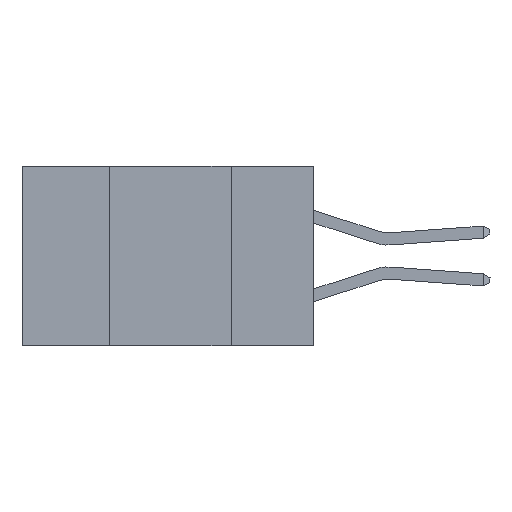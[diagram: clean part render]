
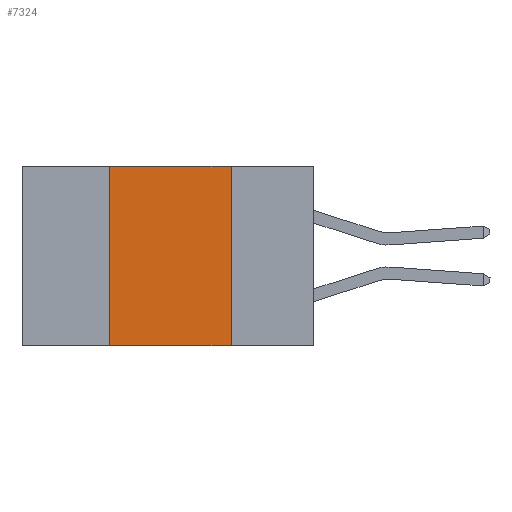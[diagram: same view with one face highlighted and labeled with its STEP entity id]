
A CAD part, left-side view. The second image highlights one B-rep face of the part: STEP entity #7324.
In plain terms, the highlighted planar face has unit normal (-1, 0, 0).
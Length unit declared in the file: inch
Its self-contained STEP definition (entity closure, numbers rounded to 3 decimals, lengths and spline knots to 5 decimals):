
#58 = CARTESIAN_POINT ( 'NONE',  ( 0., 0.42, 0. ) ) ;
#336 = CARTESIAN_POINT ( 'NONE',  ( 0., 0.42, -0.37 ) ) ;
#539 = DIRECTION ( 'NONE',  ( 0., 0., -1. ) ) ;
#818 = AXIS2_PLACEMENT_3D ( 'NONE', #9331, #6070, #539 ) ;
#955 = LINE ( 'NONE', #58, #3786 ) ;
#1066 = EDGE_CURVE ( 'NONE', #6573, #5884, #3466, .T. ) ;
#1088 = DIRECTION ( 'NONE',  ( 0., 0., 1. ) ) ;
#1171 = VERTEX_POINT ( 'NONE', #3477 ) ;
#3031 = EDGE_LOOP ( 'NONE', ( #5672, #8252, #6596, #4753 ) ) ;
#3214 = VECTOR ( 'NONE', #9567, 39.37008 ) ;
#3466 = LINE ( 'NONE', #7204, #5532 ) ;
#3477 = CARTESIAN_POINT ( 'NONE',  ( 0., 0.17, 0. ) ) ;
#3499 = DIRECTION ( 'NONE',  ( 0., -1., 0. ) ) ;
#3786 = VECTOR ( 'NONE', #1088, 39.37008 ) ;
#4381 = DIRECTION ( 'NONE',  ( 0., -1., 0. ) ) ;
#4454 = LINE ( 'NONE', #9964, #8628 ) ;
#4753 = ORIENTED_EDGE ( 'NONE', *, *, #1066, .T. ) ;
#5532 = VECTOR ( 'NONE', #3499, 39.37008 ) ;
#5593 = EDGE_CURVE ( 'NONE', #5878, #1171, #4454, .T. ) ;
#5672 = ORIENTED_EDGE ( 'NONE', *, *, #9270, .F. ) ;
#5878 = VERTEX_POINT ( 'NONE', #8434 ) ;
#5884 = VERTEX_POINT ( 'NONE', #9475 ) ;
#6070 = DIRECTION ( 'NONE',  ( 1., 0., 0. ) ) ;
#6573 = VERTEX_POINT ( 'NONE', #336 ) ;
#6596 = ORIENTED_EDGE ( 'NONE', *, *, #10728, .F. ) ;
#7204 = CARTESIAN_POINT ( 'NONE',  ( 0., 0.6, -0.37 ) ) ;
#7324 = ADVANCED_FACE ( 'NONE', ( #8849 ), #10783, .F. ) ;
#7532 = LINE ( 'NONE', #8747, #3214 ) ;
#8252 = ORIENTED_EDGE ( 'NONE', *, *, #5593, .F. ) ;
#8434 = CARTESIAN_POINT ( 'NONE',  ( 0., 0.42, 0. ) ) ;
#8628 = VECTOR ( 'NONE', #4381, 39.37008 ) ;
#8747 = CARTESIAN_POINT ( 'NONE',  ( 0., 0.17, 0. ) ) ;
#8849 = FACE_OUTER_BOUND ( 'NONE', #3031, .T. ) ;
#9270 = EDGE_CURVE ( 'NONE', #1171, #5884, #7532, .T. ) ;
#9331 = CARTESIAN_POINT ( 'NONE',  ( 0., 0.6, 0. ) ) ;
#9475 = CARTESIAN_POINT ( 'NONE',  ( 0., 0.17, -0.37 ) ) ;
#9567 = DIRECTION ( 'NONE',  ( 0., 0., -1. ) ) ;
#9964 = CARTESIAN_POINT ( 'NONE',  ( 0., 0.6, 0. ) ) ;
#10728 = EDGE_CURVE ( 'NONE', #6573, #5878, #955, .T. ) ;
#10783 = PLANE ( 'NONE',  #818 ) ;
